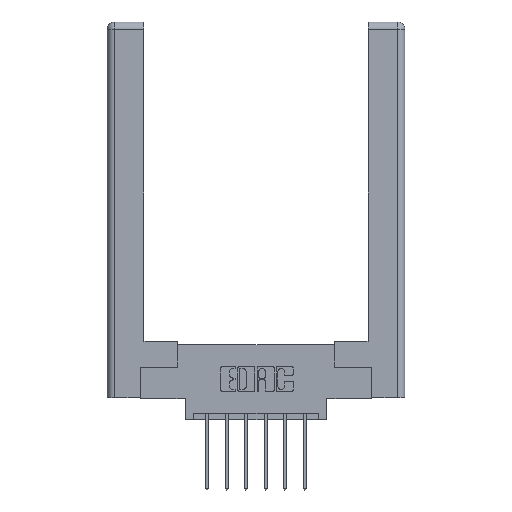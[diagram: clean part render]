
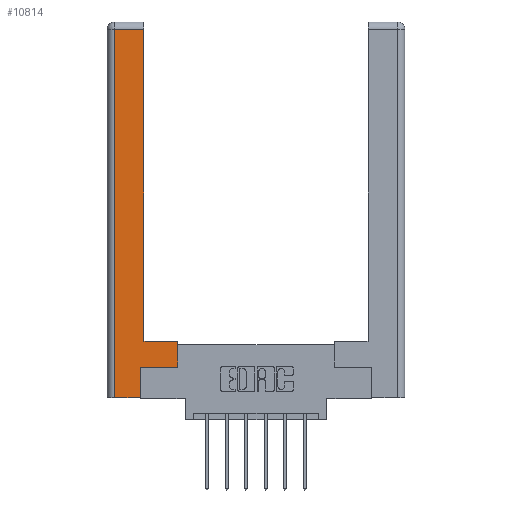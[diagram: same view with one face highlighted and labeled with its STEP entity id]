
A CAD part, top view. The second image highlights one B-rep face of the part: STEP entity #10814.
In plain terms, the highlighted planar face has unit normal (0, 0, 1).
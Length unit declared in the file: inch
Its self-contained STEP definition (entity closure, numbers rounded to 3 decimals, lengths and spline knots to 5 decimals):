
#15 = ORIENTED_EDGE ( 'NONE', *, *, #2777, .T. ) ;
#229 = VERTEX_POINT ( 'NONE', #4568 ) ;
#248 = EDGE_CURVE ( 'NONE', #4869, #9133, #2553, .T. ) ;
#419 = CARTESIAN_POINT ( 'NONE',  ( 0.565, 0.45, 0. ) ) ;
#507 = VECTOR ( 'NONE', #12057, 39.37008 ) ;
#671 = DIRECTION ( 'NONE',  ( 0., -1., 0. ) ) ;
#776 = VERTEX_POINT ( 'NONE', #5622 ) ;
#783 = FACE_OUTER_BOUND ( 'NONE', #10161, .T. ) ;
#924 = CARTESIAN_POINT ( 'NONE',  ( 0.565, 0.45, 0. ) ) ;
#1034 = CARTESIAN_POINT ( 'NONE',  ( 0.265, 0., 0. ) ) ;
#1047 = LINE ( 'NONE', #3555, #4570 ) ;
#1638 = ORIENTED_EDGE ( 'NONE', *, *, #4051, .T. ) ;
#2115 = LINE ( 'NONE', #924, #4627 ) ;
#2126 = ORIENTED_EDGE ( 'NONE', *, *, #9281, .T. ) ;
#2315 = VECTOR ( 'NONE', #11992, 39.37008 ) ;
#2327 = AXIS2_PLACEMENT_3D ( 'NONE', #4348, #10876, #2482 ) ;
#2385 = ORIENTED_EDGE ( 'NONE', *, *, #10753, .T. ) ;
#2482 = DIRECTION ( 'NONE',  ( -1., 0., 0. ) ) ;
#2553 = LINE ( 'NONE', #9130, #507 ) ;
#2683 = CARTESIAN_POINT ( 'NONE',  ( 0.0615, 0., 0. ) ) ;
#2777 = EDGE_CURVE ( 'NONE', #11202, #3501, #3683, .T. ) ;
#2845 = DIRECTION ( 'NONE',  ( 1., 0., 0. ) ) ;
#3144 = CARTESIAN_POINT ( 'NONE',  ( 0.295, 2.94, 0. ) ) ;
#3401 = PLANE ( 'NONE',  #2327 ) ;
#3444 = DIRECTION ( 'NONE',  ( -1., 0., 0. ) ) ;
#3501 = VERTEX_POINT ( 'NONE', #6402 ) ;
#3555 = CARTESIAN_POINT ( 'NONE',  ( 0.0615, 2.94, 0. ) ) ;
#3623 = ORIENTED_EDGE ( 'NONE', *, *, #4520, .T. ) ;
#3662 = VECTOR ( 'NONE', #4545, 39.37008 ) ;
#3683 = LINE ( 'NONE', #1034, #6907 ) ;
#3942 = VECTOR ( 'NONE', #671, 39.37008 ) ;
#4051 = EDGE_CURVE ( 'NONE', #229, #776, #5283, .T. ) ;
#4186 = VERTEX_POINT ( 'NONE', #3144 ) ;
#4262 = CARTESIAN_POINT ( 'NONE',  ( 0.295, 3., 0. ) ) ;
#4341 = CARTESIAN_POINT ( 'NONE',  ( 0.565, 0.245, 0. ) ) ;
#4348 = CARTESIAN_POINT ( 'NONE',  ( 0., 0., 0. ) ) ;
#4520 = EDGE_CURVE ( 'NONE', #3501, #229, #8184, .T. ) ;
#4527 = LINE ( 'NONE', #2683, #3942 ) ;
#4545 = DIRECTION ( 'NONE',  ( 1., 0., 0. ) ) ;
#4568 = CARTESIAN_POINT ( 'NONE',  ( 0.265, 0.245, 0. ) ) ;
#4570 = VECTOR ( 'NONE', #3444, 39.37008 ) ;
#4627 = VECTOR ( 'NONE', #10205, 39.37008 ) ;
#4869 = VERTEX_POINT ( 'NONE', #419 ) ;
#5085 = EDGE_CURVE ( 'NONE', #5704, #11202, #4527, .T. ) ;
#5129 = ORIENTED_EDGE ( 'NONE', *, *, #248, .T. ) ;
#5283 = LINE ( 'NONE', #4341, #3662 ) ;
#5622 = CARTESIAN_POINT ( 'NONE',  ( 0.565, 0.245, 0. ) ) ;
#5704 = VERTEX_POINT ( 'NONE', #8370 ) ;
#5750 = EDGE_CURVE ( 'NONE', #4186, #5704, #1047, .T. ) ;
#6402 = CARTESIAN_POINT ( 'NONE',  ( 0.265, 0., 0. ) ) ;
#6596 = CARTESIAN_POINT ( 'NONE',  ( 0.265, 0.245, 0. ) ) ;
#6907 = VECTOR ( 'NONE', #2845, 39.37008 ) ;
#7042 = DIRECTION ( 'NONE',  ( 0., 1., 0. ) ) ;
#7177 = CARTESIAN_POINT ( 'NONE',  ( 0.295, 0.45, 0. ) ) ;
#8184 = LINE ( 'NONE', #6596, #2315 ) ;
#8370 = CARTESIAN_POINT ( 'NONE',  ( 0.0615, 2.94, 0. ) ) ;
#8546 = LINE ( 'NONE', #4262, #12031 ) ;
#9130 = CARTESIAN_POINT ( 'NONE',  ( 0.295, 0.45, 0. ) ) ;
#9133 = VERTEX_POINT ( 'NONE', #7177 ) ;
#9281 = EDGE_CURVE ( 'NONE', #776, #4869, #2115, .T. ) ;
#10161 = EDGE_LOOP ( 'NONE', ( #2385, #12056, #11947, #15, #3623, #1638, #2126, #5129 ) ) ;
#10205 = DIRECTION ( 'NONE',  ( 0., 1., 0. ) ) ;
#10461 = CARTESIAN_POINT ( 'NONE',  ( 0.0615, 0., 0. ) ) ;
#10753 = EDGE_CURVE ( 'NONE', #9133, #4186, #8546, .T. ) ;
#10814 = ADVANCED_FACE ( 'NONE', ( #783 ), #3401, .F. ) ;
#10876 = DIRECTION ( 'NONE',  ( 0., 0., -1. ) ) ;
#11202 = VERTEX_POINT ( 'NONE', #10461 ) ;
#11947 = ORIENTED_EDGE ( 'NONE', *, *, #5085, .T. ) ;
#11992 = DIRECTION ( 'NONE',  ( 0., 1., 0. ) ) ;
#12031 = VECTOR ( 'NONE', #7042, 39.37008 ) ;
#12056 = ORIENTED_EDGE ( 'NONE', *, *, #5750, .T. ) ;
#12057 = DIRECTION ( 'NONE',  ( -1., 0., 0. ) ) ;
